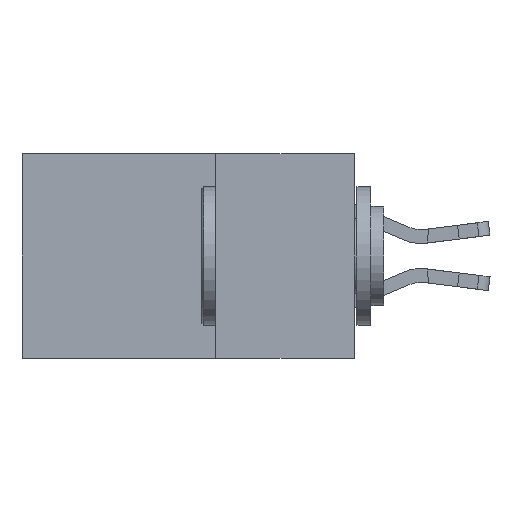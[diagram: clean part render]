
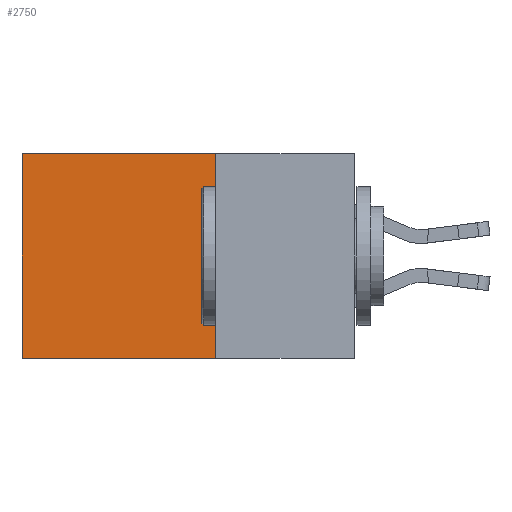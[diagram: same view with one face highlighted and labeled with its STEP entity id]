
A CAD part, left-side view. The second image highlights one B-rep face of the part: STEP entity #2750.
In plain terms, the highlighted planar face has unit normal (-1, 0, 0).
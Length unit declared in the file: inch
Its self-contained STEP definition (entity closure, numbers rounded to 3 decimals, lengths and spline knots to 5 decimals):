
#75 = LINE ( 'NONE', #3731, #2994 ) ;
#376 = EDGE_CURVE ( 'NONE', #11626, #8245, #5042, .T. ) ;
#730 = EDGE_CURVE ( 'NONE', #5606, #8245, #15753, .T. ) ;
#1184 = PLANE ( 'NONE',  #7013 ) ;
#2750 = ADVANCED_FACE ( 'NONE', ( #9374 ), #1184, .F. ) ;
#2994 = VECTOR ( 'NONE', #4491, 39.37008 ) ;
#3700 = DIRECTION ( 'NONE',  ( 0., 0., -1. ) ) ;
#3731 = CARTESIAN_POINT ( 'NONE',  ( 0.298, 0.25, 0. ) ) ;
#4491 = DIRECTION ( 'NONE',  ( 0., 1., 0. ) ) ;
#4557 = CARTESIAN_POINT ( 'NONE',  ( 0.298, 0.25, -0.37 ) ) ;
#5042 = LINE ( 'NONE', #4557, #8201 ) ;
#5532 = EDGE_CURVE ( 'NONE', #6694, #5606, #75, .T. ) ;
#5606 = VERTEX_POINT ( 'NONE', #9062 ) ;
#6455 = EDGE_CURVE ( 'NONE', #6694, #11626, #12892, .T. ) ;
#6694 = VERTEX_POINT ( 'NONE', #13831 ) ;
#7013 = AXIS2_PLACEMENT_3D ( 'NONE', #15805, #7759, #3700 ) ;
#7240 = DIRECTION ( 'NONE',  ( 0., 1., 0. ) ) ;
#7759 = DIRECTION ( 'NONE',  ( 1., 0., 0. ) ) ;
#7783 = DIRECTION ( 'NONE',  ( 0., 0., -1. ) ) ;
#7832 = VECTOR ( 'NONE', #7783, 39.37008 ) ;
#8201 = VECTOR ( 'NONE', #7240, 39.37008 ) ;
#8245 = VERTEX_POINT ( 'NONE', #11516 ) ;
#9062 = CARTESIAN_POINT ( 'NONE',  ( 0.298, 0.6, 0. ) ) ;
#9374 = FACE_OUTER_BOUND ( 'NONE', #17066, .T. ) ;
#9431 = ORIENTED_EDGE ( 'NONE', *, *, #5532, .T. ) ;
#10758 = DIRECTION ( 'NONE',  ( 0., 0., -1. ) ) ;
#11516 = CARTESIAN_POINT ( 'NONE',  ( 0.298, 0.6, -0.37 ) ) ;
#11623 = ORIENTED_EDGE ( 'NONE', *, *, #730, .T. ) ;
#11626 = VERTEX_POINT ( 'NONE', #15677 ) ;
#12324 = CARTESIAN_POINT ( 'NONE',  ( 0.298, 0.6, 0. ) ) ;
#12478 = ORIENTED_EDGE ( 'NONE', *, *, #376, .F. ) ;
#12892 = LINE ( 'NONE', #14613, #7832 ) ;
#13314 = ORIENTED_EDGE ( 'NONE', *, *, #6455, .F. ) ;
#13831 = CARTESIAN_POINT ( 'NONE',  ( 0.298, 0.25, 0. ) ) ;
#14613 = CARTESIAN_POINT ( 'NONE',  ( 0.298, 0.25, 0. ) ) ;
#14724 = VECTOR ( 'NONE', #10758, 39.37008 ) ;
#15677 = CARTESIAN_POINT ( 'NONE',  ( 0.298, 0.25, -0.37 ) ) ;
#15753 = LINE ( 'NONE', #12324, #14724 ) ;
#15805 = CARTESIAN_POINT ( 'NONE',  ( 0.298, 0.25, 0. ) ) ;
#17066 = EDGE_LOOP ( 'NONE', ( #11623, #12478, #13314, #9431 ) ) ;
